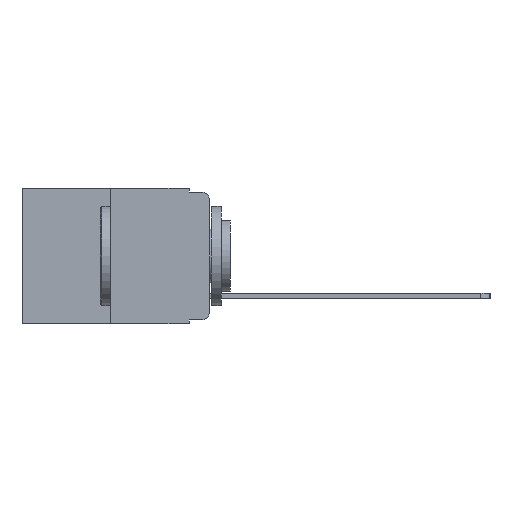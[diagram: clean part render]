
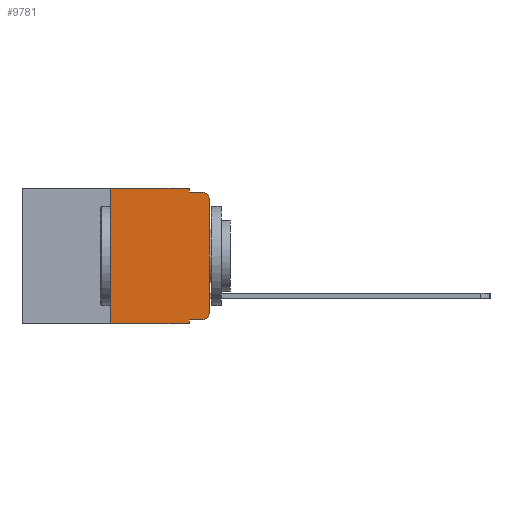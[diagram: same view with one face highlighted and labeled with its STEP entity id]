
A CAD part, left-side view. The second image highlights one B-rep face of the part: STEP entity #9781.
In plain terms, the highlighted planar face has unit normal (-1, 0, 0).
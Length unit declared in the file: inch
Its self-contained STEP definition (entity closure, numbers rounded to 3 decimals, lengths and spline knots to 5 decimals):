
#15 = CARTESIAN_POINT ( 'NONE',  ( 0., 0., 0. ) ) ;
#117 = CIRCLE ( 'NONE', #9083, 0.02 ) ;
#132 = VERTEX_POINT ( 'NONE', #256 ) ;
#164 = ORIENTED_EDGE ( 'NONE', *, *, #8883, .F. ) ;
#256 = CARTESIAN_POINT ( 'NONE',  ( 0., 0.051, 0. ) ) ;
#277 = ORIENTED_EDGE ( 'NONE', *, *, #7089, .F. ) ;
#474 = CARTESIAN_POINT ( 'NONE',  ( 0., 0.02, -0.333 ) ) ;
#479 = EDGE_CURVE ( 'NONE', #4029, #10661, #5042, .T. ) ;
#558 = DIRECTION ( 'NONE',  ( 0., 0., -1. ) ) ;
#610 = VERTEX_POINT ( 'NONE', #10202 ) ;
#1258 = LINE ( 'NONE', #10662, #3212 ) ;
#1410 = CARTESIAN_POINT ( 'NONE',  ( 0., 0.25, 0. ) ) ;
#1522 = DIRECTION ( 'NONE',  ( 0., 0., -1. ) ) ;
#1674 = CARTESIAN_POINT ( 'NONE',  ( 0., 0.051, -0.333 ) ) ;
#1964 = LINE ( 'NONE', #11042, #6693 ) ;
#2026 = CARTESIAN_POINT ( 'NONE',  ( 0., 0.02, -0.03 ) ) ;
#2088 = DIRECTION ( 'NONE',  ( 0., -1., 0. ) ) ;
#3003 = DIRECTION ( 'NONE',  ( 0., 0., -1. ) ) ;
#3212 = VECTOR ( 'NONE', #6218, 39.37008 ) ;
#3383 = EDGE_CURVE ( 'NONE', #6175, #610, #1964, .T. ) ;
#3390 = CARTESIAN_POINT ( 'NONE',  ( 0., 0.473, 0. ) ) ;
#3398 = PLANE ( 'NONE',  #6900 ) ;
#3735 = VECTOR ( 'NONE', #6219, 39.37008 ) ;
#3905 = EDGE_CURVE ( 'NONE', #6312, #4029, #5225, .T. ) ;
#3930 = CARTESIAN_POINT ( 'NONE',  ( 0., 0.051, -0.01 ) ) ;
#3958 = VECTOR ( 'NONE', #9119, 39.37008 ) ;
#3997 = VERTEX_POINT ( 'NONE', #8202 ) ;
#4029 = VERTEX_POINT ( 'NONE', #4574 ) ;
#4574 = CARTESIAN_POINT ( 'NONE',  ( 0., 0., -0.313 ) ) ;
#5042 = LINE ( 'NONE', #15, #11883 ) ;
#5131 = VERTEX_POINT ( 'NONE', #5187 ) ;
#5187 = CARTESIAN_POINT ( 'NONE',  ( 0., 0.051, -0.333 ) ) ;
#5225 = CIRCLE ( 'NONE', #11400, 0.02 ) ;
#5242 = DIRECTION ( 'NONE',  ( 0., 0., 1. ) ) ;
#5271 = LINE ( 'NONE', #10632, #5560 ) ;
#5330 = DIRECTION ( 'NONE',  ( 1., 0., 0. ) ) ;
#5560 = VECTOR ( 'NONE', #5242, 39.37008 ) ;
#5831 = EDGE_CURVE ( 'NONE', #5131, #6312, #6481, .T. ) ;
#5940 = CARTESIAN_POINT ( 'NONE',  ( 0., 0.25, -0.343 ) ) ;
#5984 = VECTOR ( 'NONE', #1522, 39.37008 ) ;
#6175 = VERTEX_POINT ( 'NONE', #5940 ) ;
#6218 = DIRECTION ( 'NONE',  ( 0., 0., -1. ) ) ;
#6219 = DIRECTION ( 'NONE',  ( 0., -1., 0. ) ) ;
#6259 = FACE_OUTER_BOUND ( 'NONE', #8931, .T. ) ;
#6279 = DIRECTION ( 'NONE',  ( -1., 0., 0. ) ) ;
#6280 = LINE ( 'NONE', #8978, #5984 ) ;
#6312 = VERTEX_POINT ( 'NONE', #474 ) ;
#6401 = VERTEX_POINT ( 'NONE', #1410 ) ;
#6481 = LINE ( 'NONE', #1674, #3958 ) ;
#6520 = CARTESIAN_POINT ( 'NONE',  ( 0., 0.051, -0.01 ) ) ;
#6693 = VECTOR ( 'NONE', #2088, 39.37008 ) ;
#6713 = ORIENTED_EDGE ( 'NONE', *, *, #10048, .T. ) ;
#6900 = AXIS2_PLACEMENT_3D ( 'NONE', #10706, #5330, #11584 ) ;
#7011 = ORIENTED_EDGE ( 'NONE', *, *, #9487, .F. ) ;
#7089 = EDGE_CURVE ( 'NONE', #5131, #610, #1258, .T. ) ;
#7724 = ORIENTED_EDGE ( 'NONE', *, *, #3383, .T. ) ;
#7867 = ORIENTED_EDGE ( 'NONE', *, *, #5831, .T. ) ;
#7874 = ORIENTED_EDGE ( 'NONE', *, *, #3905, .T. ) ;
#8070 = DIRECTION ( 'NONE',  ( 0., 0., 1. ) ) ;
#8202 = CARTESIAN_POINT ( 'NONE',  ( 0., 0.02, -0.01 ) ) ;
#8292 = EDGE_CURVE ( 'NONE', #6175, #6401, #5271, .T. ) ;
#8564 = DIRECTION ( 'NONE',  ( -1., 0., 0. ) ) ;
#8691 = LINE ( 'NONE', #3390, #3735 ) ;
#8873 = EDGE_CURVE ( 'NONE', #6401, #132, #8691, .T. ) ;
#8883 = EDGE_CURVE ( 'NONE', #132, #9940, #6280, .T. ) ;
#8931 = EDGE_LOOP ( 'NONE', ( #10070, #6713, #7011, #164, #9358, #10741, #7724, #277, #7867, #7874 ) ) ;
#8978 = CARTESIAN_POINT ( 'NONE',  ( 0., 0.051, 0. ) ) ;
#9083 = AXIS2_PLACEMENT_3D ( 'NONE', #2026, #8564, #3003 ) ;
#9084 = VECTOR ( 'NONE', #10325, 39.37008 ) ;
#9119 = DIRECTION ( 'NONE',  ( 0., -1., 0. ) ) ;
#9358 = ORIENTED_EDGE ( 'NONE', *, *, #8873, .F. ) ;
#9487 = EDGE_CURVE ( 'NONE', #9940, #3997, #11130, .T. ) ;
#9781 = ADVANCED_FACE ( 'NONE', ( #6259 ), #3398, .F. ) ;
#9940 = VERTEX_POINT ( 'NONE', #6520 ) ;
#10048 = EDGE_CURVE ( 'NONE', #10661, #3997, #117, .T. ) ;
#10070 = ORIENTED_EDGE ( 'NONE', *, *, #479, .T. ) ;
#10202 = CARTESIAN_POINT ( 'NONE',  ( 0., 0.051, -0.343 ) ) ;
#10263 = CARTESIAN_POINT ( 'NONE',  ( 0., 0., -0.03 ) ) ;
#10325 = DIRECTION ( 'NONE',  ( 0., -1., 0. ) ) ;
#10632 = CARTESIAN_POINT ( 'NONE',  ( 0., 0.25, 0. ) ) ;
#10661 = VERTEX_POINT ( 'NONE', #10263 ) ;
#10662 = CARTESIAN_POINT ( 'NONE',  ( 0., 0.051, 0. ) ) ;
#10706 = CARTESIAN_POINT ( 'NONE',  ( 0., 0.473, 0. ) ) ;
#10741 = ORIENTED_EDGE ( 'NONE', *, *, #8292, .F. ) ;
#11042 = CARTESIAN_POINT ( 'NONE',  ( 0., 0.473, -0.343 ) ) ;
#11130 = LINE ( 'NONE', #3930, #9084 ) ;
#11400 = AXIS2_PLACEMENT_3D ( 'NONE', #11598, #6279, #558 ) ;
#11584 = DIRECTION ( 'NONE',  ( 0., 0., -1. ) ) ;
#11598 = CARTESIAN_POINT ( 'NONE',  ( 0., 0.02, -0.313 ) ) ;
#11883 = VECTOR ( 'NONE', #8070, 39.37008 ) ;
